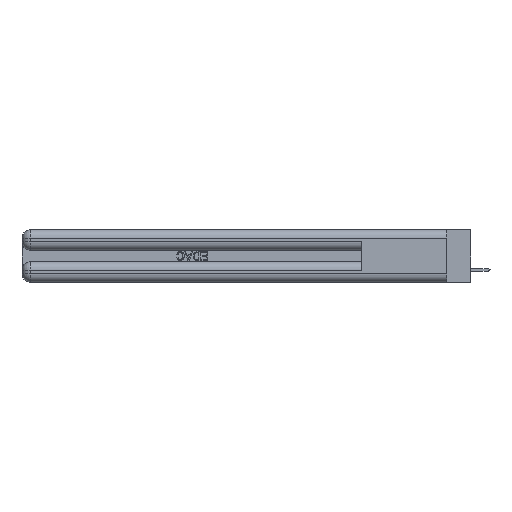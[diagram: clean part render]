
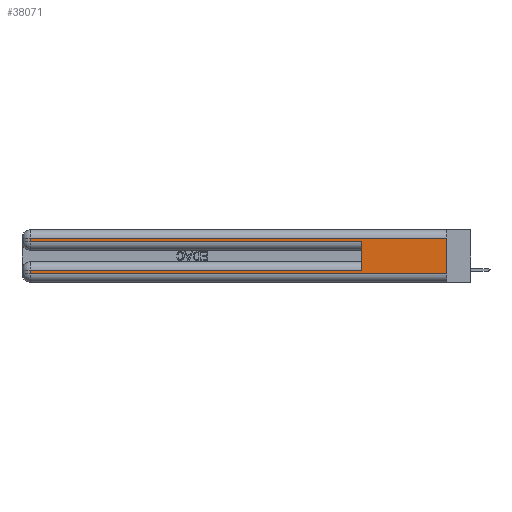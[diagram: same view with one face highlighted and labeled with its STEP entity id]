
A CAD part, left-side view. The second image highlights one B-rep face of the part: STEP entity #38071.
In plain terms, the highlighted planar face has unit normal (-1, 0, 0).
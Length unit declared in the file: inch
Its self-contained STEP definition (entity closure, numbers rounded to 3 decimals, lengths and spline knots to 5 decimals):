
#894 = ORIENTED_EDGE ( 'NONE', *, *, #27194, .F. ) ;
#911 = LINE ( 'NONE', #20146, #32587 ) ;
#1706 = CARTESIAN_POINT ( 'NONE',  ( 0., 0., 0.31 ) ) ;
#2694 = DIRECTION ( 'NONE',  ( 0., 0., -1. ) ) ;
#3405 = VERTEX_POINT ( 'NONE', #15850 ) ;
#5448 = VECTOR ( 'NONE', #15835, 39.37008 ) ;
#6287 = DIRECTION ( 'NONE',  ( 0., -1., 0. ) ) ;
#6712 = CARTESIAN_POINT ( 'NONE',  ( 0., 0., 0.085 ) ) ;
#8280 = CARTESIAN_POINT ( 'NONE',  ( 0., 0., 0.06 ) ) ;
#9002 = VECTOR ( 'NONE', #21392, 39.37008 ) ;
#10027 = EDGE_CURVE ( 'NONE', #47094, #38236, #11122, .T. ) ;
#11122 = LINE ( 'NONE', #30812, #5448 ) ;
#11138 = LINE ( 'NONE', #26356, #27916 ) ;
#11439 = CARTESIAN_POINT ( 'NONE',  ( 0., 2.94, 0.06 ) ) ;
#11513 = EDGE_CURVE ( 'NONE', #21412, #25775, #11138, .T. ) ;
#11519 = EDGE_CURVE ( 'NONE', #19857, #23761, #35910, .T. ) ;
#11660 = ORIENTED_EDGE ( 'NONE', *, *, #37206, .T. ) ;
#12225 = ORIENTED_EDGE ( 'NONE', *, *, #21697, .T. ) ;
#13539 = CARTESIAN_POINT ( 'NONE',  ( 0., 0., 0.285 ) ) ;
#13821 = ORIENTED_EDGE ( 'NONE', *, *, #11513, .F. ) ;
#14130 = DIRECTION ( 'NONE',  ( 0., 0., 1. ) ) ;
#15835 = DIRECTION ( 'NONE',  ( 0., 0., -1. ) ) ;
#15850 = CARTESIAN_POINT ( 'NONE',  ( 0., 2.94, 0.285 ) ) ;
#16558 = EDGE_CURVE ( 'NONE', #23761, #3405, #17917, .T. ) ;
#16951 = DIRECTION ( 'NONE',  ( 0., 1., 0. ) ) ;
#17917 = LINE ( 'NONE', #29143, #9002 ) ;
#18219 = CARTESIAN_POINT ( 'NONE',  ( 0., 0., 0.37 ) ) ;
#19857 = VERTEX_POINT ( 'NONE', #25673 ) ;
#20146 = CARTESIAN_POINT ( 'NONE',  ( 0., 0., 0.37 ) ) ;
#21385 = ORIENTED_EDGE ( 'NONE', *, *, #11519, .T. ) ;
#21392 = DIRECTION ( 'NONE',  ( 0., 0., -1. ) ) ;
#21412 = VERTEX_POINT ( 'NONE', #49022 ) ;
#21697 = EDGE_CURVE ( 'NONE', #3405, #25775, #32483, .T. ) ;
#23728 = LINE ( 'NONE', #8280, #26874 ) ;
#23761 = VERTEX_POINT ( 'NONE', #35878 ) ;
#25673 = CARTESIAN_POINT ( 'NONE',  ( 0., 0., 0.31 ) ) ;
#25775 = VERTEX_POINT ( 'NONE', #44141 ) ;
#26356 = CARTESIAN_POINT ( 'NONE',  ( 0., 0.6, 0.145 ) ) ;
#26661 = LINE ( 'NONE', #6712, #32747 ) ;
#26874 = VECTOR ( 'NONE', #34463, 39.37008 ) ;
#27194 = EDGE_CURVE ( 'NONE', #19857, #46650, #911, .T. ) ;
#27916 = VECTOR ( 'NONE', #14130, 39.37008 ) ;
#29143 = CARTESIAN_POINT ( 'NONE',  ( 0., 2.94, 0.37 ) ) ;
#29634 = AXIS2_PLACEMENT_3D ( 'NONE', #18219, #33420, #2694 ) ;
#29922 = DIRECTION ( 'NONE',  ( 0., 1., 0. ) ) ;
#30812 = CARTESIAN_POINT ( 'NONE',  ( 0., 2.94, 0.37 ) ) ;
#31274 = EDGE_CURVE ( 'NONE', #38236, #46650, #23728, .T. ) ;
#32479 = CARTESIAN_POINT ( 'NONE',  ( 0., 2.94, 0.085 ) ) ;
#32483 = LINE ( 'NONE', #13539, #37134 ) ;
#32587 = VECTOR ( 'NONE', #35365, 39.37008 ) ;
#32747 = VECTOR ( 'NONE', #29922, 39.37008 ) ;
#33245 = ORIENTED_EDGE ( 'NONE', *, *, #31274, .T. ) ;
#33420 = DIRECTION ( 'NONE',  ( 1., 0., 0. ) ) ;
#34264 = VECTOR ( 'NONE', #16951, 39.37008 ) ;
#34463 = DIRECTION ( 'NONE',  ( 0., -1., 0. ) ) ;
#35365 = DIRECTION ( 'NONE',  ( 0., 0., -1. ) ) ;
#35878 = CARTESIAN_POINT ( 'NONE',  ( 0., 2.94, 0.31 ) ) ;
#35910 = LINE ( 'NONE', #1706, #34264 ) ;
#37134 = VECTOR ( 'NONE', #6287, 39.37008 ) ;
#37167 = EDGE_LOOP ( 'NONE', ( #894, #21385, #47348, #12225, #13821, #11660, #39311, #33245 ) ) ;
#37206 = EDGE_CURVE ( 'NONE', #21412, #47094, #26661, .T. ) ;
#38071 = ADVANCED_FACE ( 'NONE', ( #40883 ), #48152, .F. ) ;
#38236 = VERTEX_POINT ( 'NONE', #11439 ) ;
#39311 = ORIENTED_EDGE ( 'NONE', *, *, #10027, .T. ) ;
#40269 = CARTESIAN_POINT ( 'NONE',  ( 0., 0., 0.06 ) ) ;
#40883 = FACE_OUTER_BOUND ( 'NONE', #37167, .T. ) ;
#44141 = CARTESIAN_POINT ( 'NONE',  ( 0., 0.6, 0.285 ) ) ;
#46650 = VERTEX_POINT ( 'NONE', #40269 ) ;
#47094 = VERTEX_POINT ( 'NONE', #32479 ) ;
#47348 = ORIENTED_EDGE ( 'NONE', *, *, #16558, .T. ) ;
#48152 = PLANE ( 'NONE',  #29634 ) ;
#49022 = CARTESIAN_POINT ( 'NONE',  ( 0., 0.6, 0.085 ) ) ;
